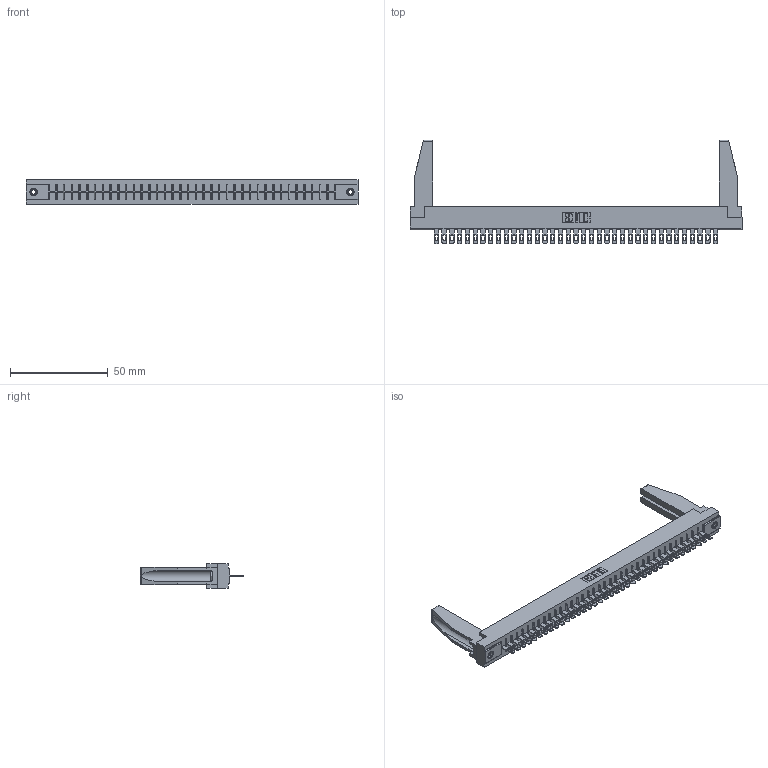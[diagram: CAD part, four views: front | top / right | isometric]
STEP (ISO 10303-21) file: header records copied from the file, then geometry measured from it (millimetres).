
FILE_DESCRIPTION (( 'STEP AP203' ), '1' );
FILE_NAME ('356-037-400-178.STEP', '2020-09-23T23:11:56', ( '' ), ( '' ), 'SwSTEP 2.0', 'SolidWorks 2020', '' );
FILE_SCHEMA (( 'CONFIG_CONTROL_DESIGN' ));
Length unit declared in the file: inch
Products named in the file (5): 306 Part_.156 Dia; 345-250-001_345-250-001-102; 356-037-400-178; 307-220-078; 306-290-001_100
Assembly tree (42 placements, depth 2):
  356-037-400-178
    306 Part_.156 Dia
    306-290-001_100  x37
    345-250-001_345-250-001-102  x2
    307-220-078  x2
Bounding box: 169.62 x 52.91 x 12.7 mm (x, y, z)
Volume: 22823.9 mm3; surface area: 23759.1 mm2
Topology: 42 solids, 42 shells, 3058 faces, 8601 edges, 5526 vertices
Faces by surface type: plane 2002, cylinder 892, sphere 148, cone 12, torus 4
Entity records: 37755 total; most frequent: CARTESIAN_POINT 6340, ORIENTED_EDGE 6244, DIRECTION 6204, EDGE_CURVE 3122, LINE 2440, VECTOR 2440, VERTEX_POINT 1976, AXIS2_PLACEMENT_3D 1882
